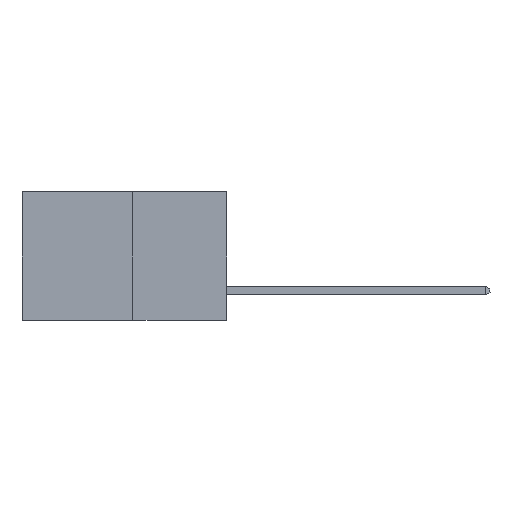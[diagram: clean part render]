
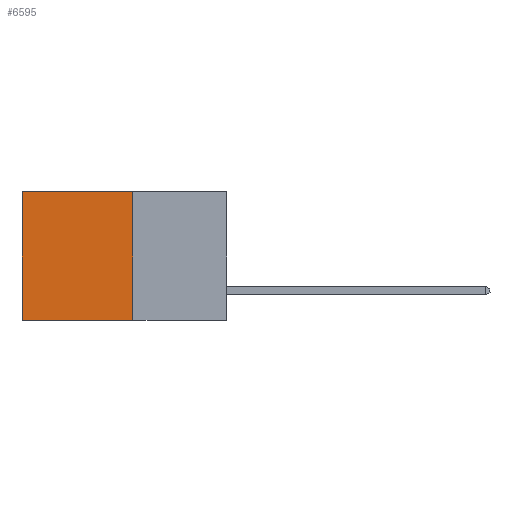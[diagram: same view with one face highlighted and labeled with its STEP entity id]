
A CAD part, left-side view. The second image highlights one B-rep face of the part: STEP entity #6595.
In plain terms, the highlighted planar face has unit normal (-1, 0, 0).
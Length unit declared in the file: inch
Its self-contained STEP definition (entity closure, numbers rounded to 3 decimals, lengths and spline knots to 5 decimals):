
#79 = CARTESIAN_POINT ( 'NONE',  ( 0.277, 0.27, -0.37 ) ) ;
#118 = CARTESIAN_POINT ( 'NONE',  ( 0.277, 0.27, -0.37 ) ) ;
#237 = ORIENTED_EDGE ( 'NONE', *, *, #1443, .T. ) ;
#353 = ORIENTED_EDGE ( 'NONE', *, *, #6563, .F. ) ;
#355 = ORIENTED_EDGE ( 'NONE', *, *, #7090, .F. ) ;
#370 = ORIENTED_EDGE ( 'NONE', *, *, #621, .T. ) ;
#496 = LINE ( 'NONE', #79, #2940 ) ;
#621 = EDGE_CURVE ( 'NONE', #1426, #851, #5214, .T. ) ;
#696 = AXIS2_PLACEMENT_3D ( 'NONE', #118, #6977, #1211 ) ;
#851 = VERTEX_POINT ( 'NONE', #6900 ) ;
#1001 = VERTEX_POINT ( 'NONE', #1746 ) ;
#1201 = EDGE_LOOP ( 'NONE', ( #237, #353, #355, #370 ) ) ;
#1211 = DIRECTION ( 'NONE',  ( 0., 0., -1. ) ) ;
#1426 = VERTEX_POINT ( 'NONE', #10381 ) ;
#1443 = EDGE_CURVE ( 'NONE', #851, #5977, #4750, .T. ) ;
#1656 = VECTOR ( 'NONE', #10355, 39.37008 ) ;
#1746 = CARTESIAN_POINT ( 'NONE',  ( 0.277, 0.27, -0.37 ) ) ;
#2940 = VECTOR ( 'NONE', #3176, 39.37008 ) ;
#3176 = DIRECTION ( 'NONE',  ( 0., 1., 0. ) ) ;
#3713 = CARTESIAN_POINT ( 'NONE',  ( 0.277, 0.59, -0.37 ) ) ;
#4750 = LINE ( 'NONE', #9407, #11645 ) ;
#5214 = LINE ( 'NONE', #11961, #10022 ) ;
#5977 = VERTEX_POINT ( 'NONE', #3713 ) ;
#6563 = EDGE_CURVE ( 'NONE', #1001, #5977, #496, .T. ) ;
#6595 = ADVANCED_FACE ( 'NONE', ( #12054 ), #10543, .F. ) ;
#6900 = CARTESIAN_POINT ( 'NONE',  ( 0.277, 0.59, 0. ) ) ;
#6977 = DIRECTION ( 'NONE',  ( 1., 0., 0. ) ) ;
#7090 = EDGE_CURVE ( 'NONE', #1426, #1001, #9183, .T. ) ;
#9183 = LINE ( 'NONE', #11207, #1656 ) ;
#9407 = CARTESIAN_POINT ( 'NONE',  ( 0.277, 0.59, -0.37 ) ) ;
#10022 = VECTOR ( 'NONE', #11820, 39.37008 ) ;
#10030 = DIRECTION ( 'NONE',  ( 0., 0., -1. ) ) ;
#10355 = DIRECTION ( 'NONE',  ( 0., 0., -1. ) ) ;
#10381 = CARTESIAN_POINT ( 'NONE',  ( 0.277, 0.27, 0. ) ) ;
#10543 = PLANE ( 'NONE',  #696 ) ;
#11207 = CARTESIAN_POINT ( 'NONE',  ( 0.277, 0.27, -0.37 ) ) ;
#11645 = VECTOR ( 'NONE', #10030, 39.37008 ) ;
#11820 = DIRECTION ( 'NONE',  ( 0., 1., 0. ) ) ;
#11961 = CARTESIAN_POINT ( 'NONE',  ( 0.277, 0.27, 0. ) ) ;
#12054 = FACE_OUTER_BOUND ( 'NONE', #1201, .T. ) ;
